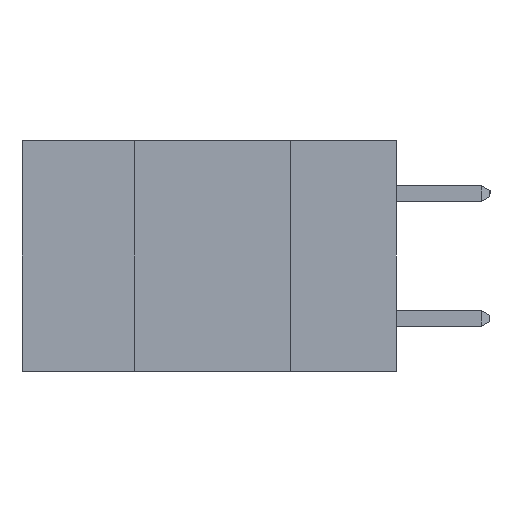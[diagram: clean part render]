
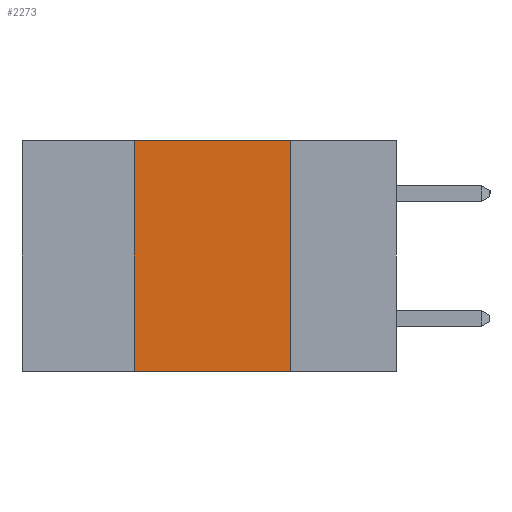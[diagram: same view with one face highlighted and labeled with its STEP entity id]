
A CAD part, left-side view. The second image highlights one B-rep face of the part: STEP entity #2273.
In plain terms, the highlighted planar face has unit normal (-1, 0, 0).
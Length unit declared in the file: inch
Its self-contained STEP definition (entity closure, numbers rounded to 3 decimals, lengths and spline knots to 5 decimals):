
#8 = DIRECTION ( 'NONE',  ( 0., -1., 0. ) ) ;
#66 = DIRECTION ( 'NONE',  ( 0., 0., -1. ) ) ;
#176 = EDGE_CURVE ( 'NONE', #719, #2476, #3095, .T. ) ;
#485 = ORIENTED_EDGE ( 'NONE', *, *, #1038, .F. ) ;
#719 = VERTEX_POINT ( 'NONE', #8668 ) ;
#771 = DIRECTION ( 'NONE',  ( 0., -1., 0. ) ) ;
#818 = DIRECTION ( 'NONE',  ( 0., 0., 1. ) ) ;
#951 = ORIENTED_EDGE ( 'NONE', *, *, #176, .F. ) ;
#1038 = EDGE_CURVE ( 'NONE', #7239, #4072, #4522, .T. ) ;
#1235 = ORIENTED_EDGE ( 'NONE', *, *, #9270, .F. ) ;
#1460 = CARTESIAN_POINT ( 'NONE',  ( 0., 0.6, 0. ) ) ;
#1505 = DIRECTION ( 'NONE',  ( 0., 0., -1. ) ) ;
#1742 = CARTESIAN_POINT ( 'NONE',  ( 0., 0.42, -0.37 ) ) ;
#2016 = CARTESIAN_POINT ( 'NONE',  ( 0., 0.42, 0. ) ) ;
#2120 = CARTESIAN_POINT ( 'NONE',  ( 0., 0.17, -0.37 ) ) ;
#2233 = LINE ( 'NONE', #5282, #8755 ) ;
#2273 = ADVANCED_FACE ( 'NONE', ( #9714 ), #8291, .F. ) ;
#2376 = VECTOR ( 'NONE', #818, 39.37008 ) ;
#2476 = VERTEX_POINT ( 'NONE', #2016 ) ;
#3013 = EDGE_LOOP ( 'NONE', ( #485, #1235, #951, #7033 ) ) ;
#3095 = LINE ( 'NONE', #1742, #2376 ) ;
#3106 = CARTESIAN_POINT ( 'NONE',  ( 0., 0.6, -0.37 ) ) ;
#4072 = VERTEX_POINT ( 'NONE', #2120 ) ;
#4476 = LINE ( 'NONE', #3106, #5426 ) ;
#4522 = LINE ( 'NONE', #8289, #9081 ) ;
#5282 = CARTESIAN_POINT ( 'NONE',  ( 0., 0.6, 0. ) ) ;
#5426 = VECTOR ( 'NONE', #771, 39.37008 ) ;
#5833 = AXIS2_PLACEMENT_3D ( 'NONE', #1460, #8927, #1505 ) ;
#7033 = ORIENTED_EDGE ( 'NONE', *, *, #7214, .T. ) ;
#7214 = EDGE_CURVE ( 'NONE', #719, #4072, #4476, .T. ) ;
#7239 = VERTEX_POINT ( 'NONE', #9012 ) ;
#8289 = CARTESIAN_POINT ( 'NONE',  ( 0., 0.17, -0.37 ) ) ;
#8291 = PLANE ( 'NONE',  #5833 ) ;
#8668 = CARTESIAN_POINT ( 'NONE',  ( 0., 0.42, -0.37 ) ) ;
#8755 = VECTOR ( 'NONE', #8, 39.37008 ) ;
#8927 = DIRECTION ( 'NONE',  ( 1., 0., 0. ) ) ;
#9012 = CARTESIAN_POINT ( 'NONE',  ( 0., 0.17, 0. ) ) ;
#9081 = VECTOR ( 'NONE', #66, 39.37008 ) ;
#9270 = EDGE_CURVE ( 'NONE', #2476, #7239, #2233, .T. ) ;
#9714 = FACE_OUTER_BOUND ( 'NONE', #3013, .T. ) ;
